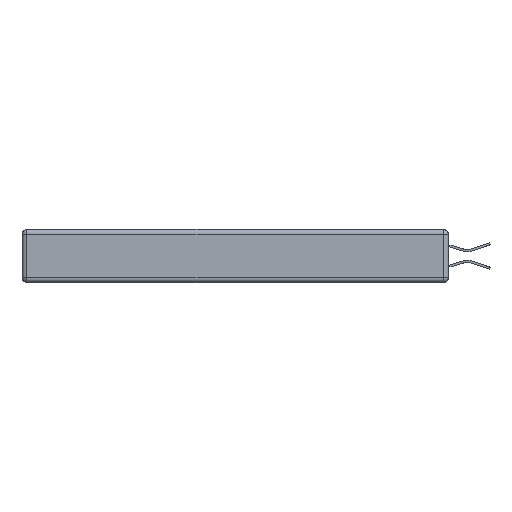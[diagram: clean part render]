
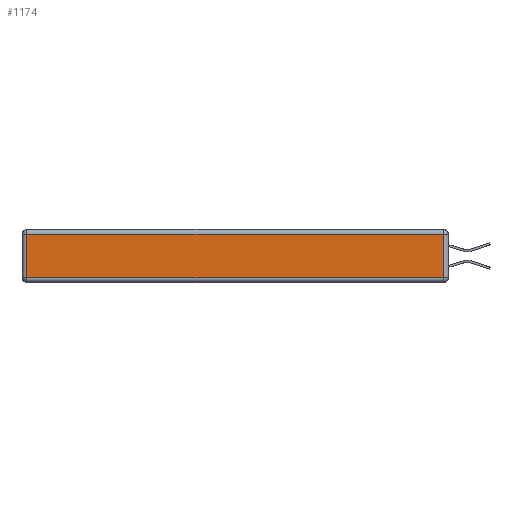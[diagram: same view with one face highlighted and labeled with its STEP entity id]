
A CAD part, left-side view. The second image highlights one B-rep face of the part: STEP entity #1174.
In plain terms, the highlighted planar face has unit normal (-1, 0, 0).
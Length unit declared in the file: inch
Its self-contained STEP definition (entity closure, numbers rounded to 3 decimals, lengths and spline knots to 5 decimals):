
#1174 = ADVANCED_FACE ( 'NONE', ( #23689 ), #13068, .T. ) ;
#4031 = EDGE_CURVE ( 'NONE', #18886, #19771, #9300, .T. ) ;
#5584 = CARTESIAN_POINT ( 'NONE',  ( 0., 2.72, -0.313 ) ) ;
#6292 = VERTEX_POINT ( 'NONE', #5584 ) ;
#6505 = VECTOR ( 'NONE', #15503, 39.37008 ) ;
#8473 = VECTOR ( 'NONE', #11398, 39.37008 ) ;
#8951 = ORIENTED_EDGE ( 'NONE', *, *, #13312, .T. ) ;
#9300 = LINE ( 'NONE', #33495, #6505 ) ;
#10698 = EDGE_CURVE ( 'NONE', #25319, #6292, #32787, .T. ) ;
#11048 = DIRECTION ( 'NONE',  ( 0., 1., 0. ) ) ;
#11277 = CARTESIAN_POINT ( 'NONE',  ( 0., 2.75, -0.03 ) ) ;
#11398 = DIRECTION ( 'NONE',  ( 0., -1., 0. ) ) ;
#13068 = PLANE ( 'NONE',  #14711 ) ;
#13312 = EDGE_CURVE ( 'NONE', #19771, #25319, #15939, .T. ) ;
#13343 = LINE ( 'NONE', #16399, #8473 ) ;
#14191 = ORIENTED_EDGE ( 'NONE', *, *, #4031, .T. ) ;
#14711 = AXIS2_PLACEMENT_3D ( 'NONE', #15677, #18595, #21567 ) ;
#15503 = DIRECTION ( 'NONE',  ( 0., 0., 1. ) ) ;
#15677 = CARTESIAN_POINT ( 'NONE',  ( 0., 0., -0.343 ) ) ;
#15939 = LINE ( 'NONE', #11277, #23647 ) ;
#16243 = ORIENTED_EDGE ( 'NONE', *, *, #26459, .T. ) ;
#16399 = CARTESIAN_POINT ( 'NONE',  ( 0., 0., -0.313 ) ) ;
#16953 = CARTESIAN_POINT ( 'NONE',  ( 0., 0.03, -0.313 ) ) ;
#18595 = DIRECTION ( 'NONE',  ( -1., 0., 0. ) ) ;
#18886 = VERTEX_POINT ( 'NONE', #16953 ) ;
#19771 = VERTEX_POINT ( 'NONE', #20889 ) ;
#20889 = CARTESIAN_POINT ( 'NONE',  ( 0., 0.03, -0.03 ) ) ;
#21567 = DIRECTION ( 'NONE',  ( 0., 0., 1. ) ) ;
#22570 = DIRECTION ( 'NONE',  ( 0., 0., -1. ) ) ;
#23647 = VECTOR ( 'NONE', #11048, 39.37008 ) ;
#23689 = FACE_OUTER_BOUND ( 'NONE', #29236, .T. ) ;
#25319 = VERTEX_POINT ( 'NONE', #29386 ) ;
#26459 = EDGE_CURVE ( 'NONE', #6292, #18886, #13343, .T. ) ;
#27912 = VECTOR ( 'NONE', #22570, 39.37008 ) ;
#29236 = EDGE_LOOP ( 'NONE', ( #16243, #14191, #8951, #33093 ) ) ;
#29386 = CARTESIAN_POINT ( 'NONE',  ( 0., 2.72, -0.03 ) ) ;
#32662 = CARTESIAN_POINT ( 'NONE',  ( 0., 2.72, -0.343 ) ) ;
#32787 = LINE ( 'NONE', #32662, #27912 ) ;
#33093 = ORIENTED_EDGE ( 'NONE', *, *, #10698, .T. ) ;
#33495 = CARTESIAN_POINT ( 'NONE',  ( 0., 0.03, -0.343 ) ) ;
